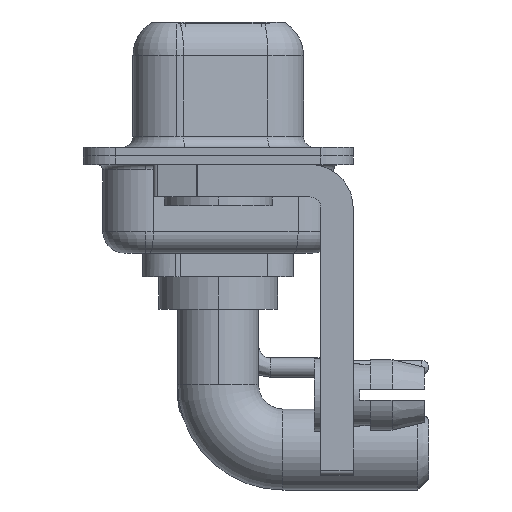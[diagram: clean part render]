
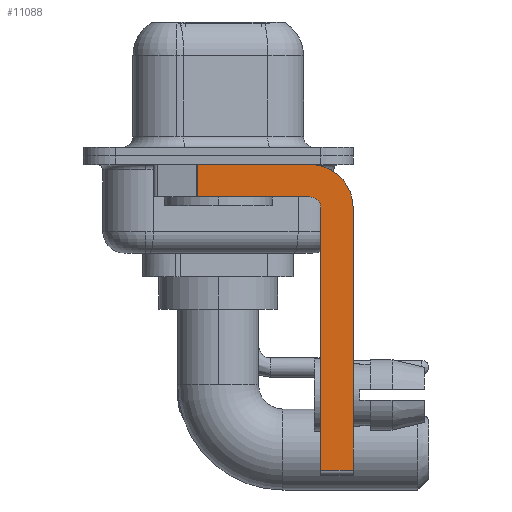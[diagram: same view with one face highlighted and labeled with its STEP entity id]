
A CAD part, left-side view. The second image highlights one B-rep face of the part: STEP entity #11088.
In plain terms, the highlighted planar face has unit normal (-1, 0, 0).
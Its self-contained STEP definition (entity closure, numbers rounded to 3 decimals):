
#151 = ORIENTED_EDGE ( 'NONE', *, *, #18250, .F. ) ;
#240 = PLANE ( 'NONE',  #17751 ) ;
#517 = CARTESIAN_POINT ( 'NONE',  ( -2.9, -4.75, -14.8 ) ) ;
#1084 = VECTOR ( 'NONE', #3489, 1000. ) ;
#1322 = CARTESIAN_POINT ( 'NONE',  ( -2.9, -4.25, -0.4 ) ) ;
#1494 = VERTEX_POINT ( 'NONE', #1322 ) ;
#1928 = LINE ( 'NONE', #517, #11709 ) ;
#2042 = DIRECTION ( 'NONE',  ( 0., 0., 1. ) ) ;
#2184 = CIRCLE ( 'NONE', #15839, 2. ) ;
#2296 = VERTEX_POINT ( 'NONE', #17106 ) ;
#2443 = LINE ( 'NONE', #7120, #3032 ) ;
#2528 = CARTESIAN_POINT ( 'NONE',  ( -2.9, -4.75, -14.55 ) ) ;
#2684 = ORIENTED_EDGE ( 'NONE', *, *, #8269, .F. ) ;
#2783 = DIRECTION ( 'NONE',  ( 0., 0., -1. ) ) ;
#3032 = VECTOR ( 'NONE', #10216, 1000. ) ;
#3428 = CARTESIAN_POINT ( 'NONE',  ( -2.9, 3., -0.4 ) ) ;
#3489 = DIRECTION ( 'NONE',  ( 0., -1., 0. ) ) ;
#3873 = LINE ( 'NONE', #5565, #10673 ) ;
#4504 = VERTEX_POINT ( 'NONE', #2528 ) ;
#5565 = CARTESIAN_POINT ( 'NONE',  ( -2.9, -4.25, -1.9 ) ) ;
#5699 = ORIENTED_EDGE ( 'NONE', *, *, #18664, .F. ) ;
#5986 = DIRECTION ( 'NONE',  ( 1., 0., 0. ) ) ;
#5993 = ORIENTED_EDGE ( 'NONE', *, *, #6982, .T. ) ;
#6982 = EDGE_CURVE ( 'NONE', #16166, #15474, #19179, .T. ) ;
#7120 = CARTESIAN_POINT ( 'NONE',  ( -2.9, -6.25, -2.4 ) ) ;
#7258 = VECTOR ( 'NONE', #14084, 1000. ) ;
#7524 = EDGE_CURVE ( 'NONE', #4504, #8701, #9360, .T. ) ;
#7647 = CARTESIAN_POINT ( 'NONE',  ( -2.9, 0.978, -1.9 ) ) ;
#7970 = CARTESIAN_POINT ( 'NONE',  ( -2.9, -4.25, -14.55 ) ) ;
#8205 = DIRECTION ( 'NONE',  ( 0., 0., -1. ) ) ;
#8269 = EDGE_CURVE ( 'NONE', #2296, #15474, #3873, .T. ) ;
#8339 = CARTESIAN_POINT ( 'NONE',  ( -2.9, -6.25, -14.55 ) ) ;
#8701 = VERTEX_POINT ( 'NONE', #8339 ) ;
#8752 = CARTESIAN_POINT ( 'NONE',  ( -2.9, 0.978, -1.9 ) ) ;
#9360 = LINE ( 'NONE', #7970, #1084 ) ;
#9596 = DIRECTION ( 'NONE',  ( 1., 0., 0. ) ) ;
#9612 = DIRECTION ( 'NONE',  ( -1., 0., 0. ) ) ;
#10216 = DIRECTION ( 'NONE',  ( 0., 0., -1. ) ) ;
#10403 = EDGE_CURVE ( 'NONE', #14461, #2296, #10416, .T. ) ;
#10416 = CIRCLE ( 'NONE', #18674, 0.5 ) ;
#10673 = VECTOR ( 'NONE', #11642, 1000. ) ;
#10788 = CARTESIAN_POINT ( 'NONE',  ( -2.9, 0.978, -0.4 ) ) ;
#11088 = ADVANCED_FACE ( 'NONE', ( #12601 ), #240, .F. ) ;
#11167 = EDGE_CURVE ( 'NONE', #16166, #1494, #17051, .T. ) ;
#11581 = CARTESIAN_POINT ( 'NONE',  ( -2.9, -6.25, -2.4 ) ) ;
#11642 = DIRECTION ( 'NONE',  ( 0., 1., 0. ) ) ;
#11709 = VECTOR ( 'NONE', #15555, 1000. ) ;
#11904 = EDGE_LOOP ( 'NONE', ( #14771, #5993, #2684, #16575, #151, #18308, #13693, #5699 ) ) ;
#12220 = VECTOR ( 'NONE', #2783, 1000. ) ;
#12601 = FACE_OUTER_BOUND ( 'NONE', #11904, .T. ) ;
#13693 = ORIENTED_EDGE ( 'NONE', *, *, #15731, .F. ) ;
#14084 = DIRECTION ( 'NONE',  ( 0., -1., 0. ) ) ;
#14461 = VERTEX_POINT ( 'NONE', #19633 ) ;
#14771 = ORIENTED_EDGE ( 'NONE', *, *, #11167, .F. ) ;
#14786 = VERTEX_POINT ( 'NONE', #11581 ) ;
#15474 = VERTEX_POINT ( 'NONE', #7647 ) ;
#15555 = DIRECTION ( 'NONE',  ( 0., 0., 1. ) ) ;
#15586 = CARTESIAN_POINT ( 'NONE',  ( -2.9, -4.25, -2.4 ) ) ;
#15651 = CARTESIAN_POINT ( 'NONE',  ( -2.9, -4.25, -2.4 ) ) ;
#15731 = EDGE_CURVE ( 'NONE', #14786, #8701, #2443, .T. ) ;
#15839 = AXIS2_PLACEMENT_3D ( 'NONE', #19600, #5986, #18605 ) ;
#16166 = VERTEX_POINT ( 'NONE', #10788 ) ;
#16575 = ORIENTED_EDGE ( 'NONE', *, *, #10403, .F. ) ;
#17051 = LINE ( 'NONE', #3428, #7258 ) ;
#17106 = CARTESIAN_POINT ( 'NONE',  ( -2.9, -4.25, -1.9 ) ) ;
#17751 = AXIS2_PLACEMENT_3D ( 'NONE', #15651, #9596, #8205 ) ;
#18250 = EDGE_CURVE ( 'NONE', #4504, #14461, #1928, .T. ) ;
#18308 = ORIENTED_EDGE ( 'NONE', *, *, #7524, .T. ) ;
#18605 = DIRECTION ( 'NONE',  ( 0., 0., -1. ) ) ;
#18664 = EDGE_CURVE ( 'NONE', #1494, #14786, #2184, .T. ) ;
#18674 = AXIS2_PLACEMENT_3D ( 'NONE', #15586, #9612, #2042 ) ;
#19179 = LINE ( 'NONE', #8752, #12220 ) ;
#19600 = CARTESIAN_POINT ( 'NONE',  ( -2.9, -4.25, -2.4 ) ) ;
#19633 = CARTESIAN_POINT ( 'NONE',  ( -2.9, -4.75, -2.4 ) ) ;
